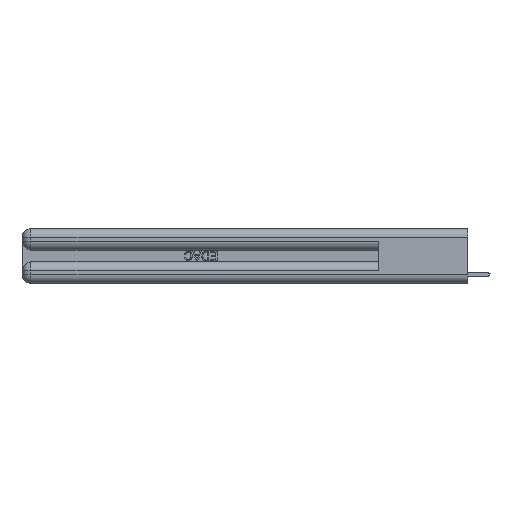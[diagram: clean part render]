
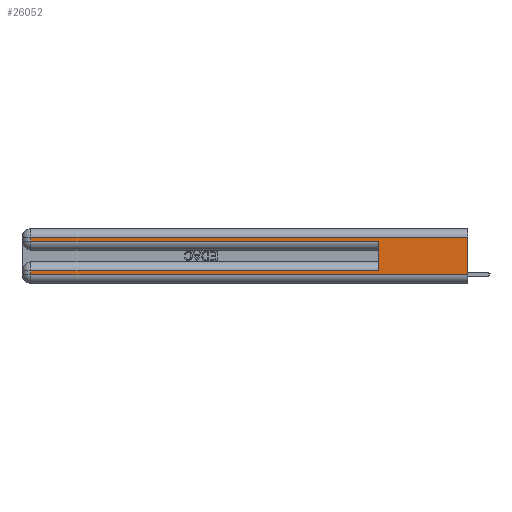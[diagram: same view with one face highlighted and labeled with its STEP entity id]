
A CAD part, left-side view. The second image highlights one B-rep face of the part: STEP entity #26052.
In plain terms, the highlighted planar face has unit normal (-1, 0, 0).
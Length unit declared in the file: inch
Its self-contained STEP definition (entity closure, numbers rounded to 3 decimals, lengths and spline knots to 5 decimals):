
#239 = EDGE_CURVE ( 'NONE', #13009, #25690, #24687, .T. ) ;
#392 = VERTEX_POINT ( 'NONE', #19441 ) ;
#573 = CARTESIAN_POINT ( 'NONE',  ( 0., 2.94, 0.285 ) ) ;
#709 = CARTESIAN_POINT ( 'NONE',  ( 0., 2.94, 0.085 ) ) ;
#1355 = EDGE_CURVE ( 'NONE', #392, #13988, #21015, .T. ) ;
#1530 = VECTOR ( 'NONE', #7009, 39.37008 ) ;
#1687 = LINE ( 'NONE', #2993, #28801 ) ;
#2991 = ORIENTED_EDGE ( 'NONE', *, *, #8444, .T. ) ;
#2993 = CARTESIAN_POINT ( 'NONE',  ( 0., 2.94, 0.37 ) ) ;
#3482 = VECTOR ( 'NONE', #9120, 39.37008 ) ;
#3758 = CARTESIAN_POINT ( 'NONE',  ( 0., 2.94, 0.31 ) ) ;
#3784 = VECTOR ( 'NONE', #5578, 39.37008 ) ;
#4121 = EDGE_CURVE ( 'NONE', #18220, #6642, #1687, .T. ) ;
#4493 = CARTESIAN_POINT ( 'NONE',  ( 0., 0., 0.285 ) ) ;
#4634 = PLANE ( 'NONE',  #7788 ) ;
#5152 = EDGE_CURVE ( 'NONE', #13009, #18220, #24005, .T. ) ;
#5578 = DIRECTION ( 'NONE',  ( 0., 1., 0. ) ) ;
#5603 = LINE ( 'NONE', #12591, #3784 ) ;
#6569 = DIRECTION ( 'NONE',  ( 0., -1., 0. ) ) ;
#6642 = VERTEX_POINT ( 'NONE', #25597 ) ;
#6777 = VECTOR ( 'NONE', #7892, 39.37008 ) ;
#7009 = DIRECTION ( 'NONE',  ( 0., 0., -1. ) ) ;
#7788 = AXIS2_PLACEMENT_3D ( 'NONE', #14002, #9415, #11570 ) ;
#7892 = DIRECTION ( 'NONE',  ( 0., 1., 0. ) ) ;
#8444 = EDGE_CURVE ( 'NONE', #11857, #30160, #26405, .T. ) ;
#8726 = ORIENTED_EDGE ( 'NONE', *, *, #4121, .T. ) ;
#8903 = DIRECTION ( 'NONE',  ( 0., 0., -1. ) ) ;
#9120 = DIRECTION ( 'NONE',  ( 0., -1., 0. ) ) ;
#9415 = DIRECTION ( 'NONE',  ( 1., 0., 0. ) ) ;
#9780 = EDGE_CURVE ( 'NONE', #30160, #25690, #11477, .T. ) ;
#10081 = ORIENTED_EDGE ( 'NONE', *, *, #14232, .T. ) ;
#10129 = LINE ( 'NONE', #23246, #3482 ) ;
#10381 = CARTESIAN_POINT ( 'NONE',  ( 0., 0., 0.06 ) ) ;
#11477 = LINE ( 'NONE', #4493, #20651 ) ;
#11570 = DIRECTION ( 'NONE',  ( 0., 0., -1. ) ) ;
#11857 = VERTEX_POINT ( 'NONE', #3758 ) ;
#12591 = CARTESIAN_POINT ( 'NONE',  ( 0., 0., 0.31 ) ) ;
#12630 = VECTOR ( 'NONE', #13246, 39.37008 ) ;
#13009 = VERTEX_POINT ( 'NONE', #20848 ) ;
#13246 = DIRECTION ( 'NONE',  ( 0., 0., 1. ) ) ;
#13958 = VECTOR ( 'NONE', #8903, 39.37008 ) ;
#13988 = VERTEX_POINT ( 'NONE', #10381 ) ;
#14002 = CARTESIAN_POINT ( 'NONE',  ( 0., 0., 0.37 ) ) ;
#14232 = EDGE_CURVE ( 'NONE', #6642, #13988, #10129, .T. ) ;
#15210 = FACE_OUTER_BOUND ( 'NONE', #15305, .T. ) ;
#15305 = EDGE_LOOP ( 'NONE', ( #30186, #24927, #2991, #16232, #17786, #21852, #8726, #10081 ) ) ;
#15488 = EDGE_CURVE ( 'NONE', #392, #11857, #5603, .T. ) ;
#16232 = ORIENTED_EDGE ( 'NONE', *, *, #9780, .T. ) ;
#17196 = CARTESIAN_POINT ( 'NONE',  ( 0., 0., 0.085 ) ) ;
#17758 = CARTESIAN_POINT ( 'NONE',  ( 0., 0.6, 0.145 ) ) ;
#17786 = ORIENTED_EDGE ( 'NONE', *, *, #239, .F. ) ;
#18220 = VERTEX_POINT ( 'NONE', #709 ) ;
#19441 = CARTESIAN_POINT ( 'NONE',  ( 0., 0., 0.31 ) ) ;
#20651 = VECTOR ( 'NONE', #6569, 39.37008 ) ;
#20848 = CARTESIAN_POINT ( 'NONE',  ( 0., 0.6, 0.085 ) ) ;
#20865 = CARTESIAN_POINT ( 'NONE',  ( 0., 0.6, 0.285 ) ) ;
#21015 = LINE ( 'NONE', #30109, #1530 ) ;
#21852 = ORIENTED_EDGE ( 'NONE', *, *, #5152, .T. ) ;
#23246 = CARTESIAN_POINT ( 'NONE',  ( 0., 0., 0.06 ) ) ;
#24005 = LINE ( 'NONE', #17196, #6777 ) ;
#24687 = LINE ( 'NONE', #17758, #12630 ) ;
#24927 = ORIENTED_EDGE ( 'NONE', *, *, #15488, .T. ) ;
#25597 = CARTESIAN_POINT ( 'NONE',  ( 0., 2.94, 0.06 ) ) ;
#25690 = VERTEX_POINT ( 'NONE', #20865 ) ;
#26052 = ADVANCED_FACE ( 'NONE', ( #15210 ), #4634, .F. ) ;
#26405 = LINE ( 'NONE', #27810, #13958 ) ;
#27810 = CARTESIAN_POINT ( 'NONE',  ( 0., 2.94, 0.37 ) ) ;
#28801 = VECTOR ( 'NONE', #28873, 39.37008 ) ;
#28873 = DIRECTION ( 'NONE',  ( 0., 0., -1. ) ) ;
#30109 = CARTESIAN_POINT ( 'NONE',  ( 0., 0., 0.37 ) ) ;
#30160 = VERTEX_POINT ( 'NONE', #573 ) ;
#30186 = ORIENTED_EDGE ( 'NONE', *, *, #1355, .F. ) ;
